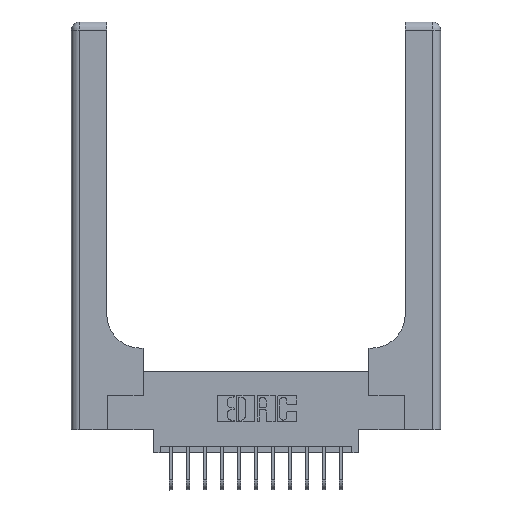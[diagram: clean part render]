
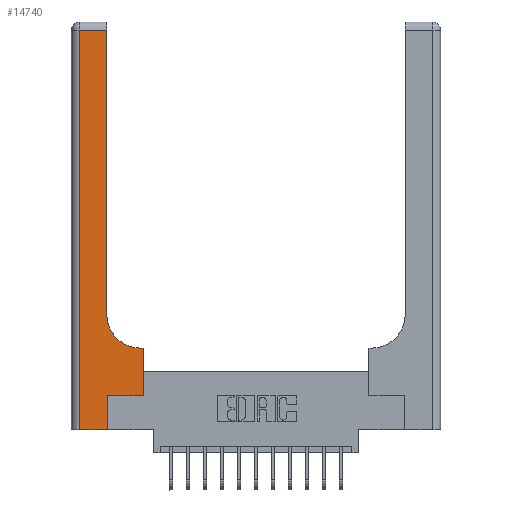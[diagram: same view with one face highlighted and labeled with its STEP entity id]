
A CAD part, top view. The second image highlights one B-rep face of the part: STEP entity #14740.
In plain terms, the highlighted planar face has unit normal (0, 0, 1).
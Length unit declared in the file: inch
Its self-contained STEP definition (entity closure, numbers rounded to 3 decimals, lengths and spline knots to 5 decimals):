
#79 = DIRECTION ( 'NONE',  ( 1., 0., 0. ) ) ;
#195 = VERTEX_POINT ( 'NONE', #12885 ) ;
#504 = CARTESIAN_POINT ( 'NONE',  ( 0.06, 3., 0.37 ) ) ;
#670 = CIRCLE ( 'NONE', #18062, 0.25 ) ;
#722 = VERTEX_POINT ( 'NONE', #9341 ) ;
#1000 = CARTESIAN_POINT ( 'NONE',  ( 0.51, 0.85, 0.37 ) ) ;
#1031 = DIRECTION ( 'NONE',  ( 0., 0., -1. ) ) ;
#1051 = LINE ( 'NONE', #11383, #17765 ) ;
#1323 = DIRECTION ( 'NONE',  ( 0., 1., 0. ) ) ;
#1368 = DIRECTION ( 'NONE',  ( 0., 0., -1. ) ) ;
#1375 = EDGE_CURVE ( 'NONE', #17372, #10682, #7767, .T. ) ;
#1478 = ORIENTED_EDGE ( 'NONE', *, *, #1375, .T. ) ;
#2265 = PLANE ( 'NONE',  #11930 ) ;
#2561 = ORIENTED_EDGE ( 'NONE', *, *, #18293, .T. ) ;
#2565 = CARTESIAN_POINT ( 'NONE',  ( 0.26, 3., 0.37 ) ) ;
#2668 = CARTESIAN_POINT ( 'NONE',  ( 0.265, 0., 0.37 ) ) ;
#2794 = CARTESIAN_POINT ( 'NONE',  ( 0.06, 2.94, 0.37 ) ) ;
#3109 = EDGE_CURVE ( 'NONE', #13241, #4829, #8973, .T. ) ;
#3165 = DIRECTION ( 'NONE',  ( -1., 0., 0. ) ) ;
#3443 = ORIENTED_EDGE ( 'NONE', *, *, #16912, .T. ) ;
#3527 = FACE_OUTER_BOUND ( 'NONE', #12988, .T. ) ;
#4707 = EDGE_CURVE ( 'NONE', #9349, #17372, #6609, .T. ) ;
#4770 = VERTEX_POINT ( 'NONE', #13927 ) ;
#4829 = VERTEX_POINT ( 'NONE', #18791 ) ;
#4986 = ORIENTED_EDGE ( 'NONE', *, *, #4707, .T. ) ;
#6500 = DIRECTION ( 'NONE',  ( -1., 0., 0. ) ) ;
#6508 = CARTESIAN_POINT ( 'NONE',  ( 0.265, 0., 0.37 ) ) ;
#6609 = LINE ( 'NONE', #2565, #9350 ) ;
#6791 = CARTESIAN_POINT ( 'NONE',  ( 0., 3., 0.37 ) ) ;
#7500 = CARTESIAN_POINT ( 'NONE',  ( 0.265, 0.25, 0.37 ) ) ;
#7767 = LINE ( 'NONE', #16255, #10397 ) ;
#7913 = CARTESIAN_POINT ( 'NONE',  ( 0., 0., 0.37 ) ) ;
#8245 = CARTESIAN_POINT ( 'NONE',  ( 0.26, 0.85, 0.37 ) ) ;
#8683 = LINE ( 'NONE', #6508, #18330 ) ;
#8973 = LINE ( 'NONE', #11668, #12826 ) ;
#9188 = ORIENTED_EDGE ( 'NONE', *, *, #16357, .T. ) ;
#9341 = CARTESIAN_POINT ( 'NONE',  ( 0.06, 0., 0.37 ) ) ;
#9349 = VERTEX_POINT ( 'NONE', #8245 ) ;
#9350 = VECTOR ( 'NONE', #17087, 39.37008 ) ;
#9550 = DIRECTION ( 'NONE',  ( 0., 1., 0. ) ) ;
#9729 = DIRECTION ( 'NONE',  ( 1., 0., 0. ) ) ;
#9775 = ORIENTED_EDGE ( 'NONE', *, *, #14825, .T. ) ;
#9786 = EDGE_CURVE ( 'NONE', #195, #4770, #13342, .T. ) ;
#10045 = VECTOR ( 'NONE', #17557, 39.37008 ) ;
#10397 = VECTOR ( 'NONE', #3165, 39.37008 ) ;
#10682 = VERTEX_POINT ( 'NONE', #2794 ) ;
#10752 = LINE ( 'NONE', #504, #17469 ) ;
#10783 = LINE ( 'NONE', #7913, #15305 ) ;
#11383 = CARTESIAN_POINT ( 'NONE',  ( 0.528, 0.25, 0.37 ) ) ;
#11668 = CARTESIAN_POINT ( 'NONE',  ( 0.265, 0.25, 0.37 ) ) ;
#11930 = AXIS2_PLACEMENT_3D ( 'NONE', #6791, #1031, #6500 ) ;
#12074 = CARTESIAN_POINT ( 'NONE',  ( 0.26, 2.94, 0.37 ) ) ;
#12739 = ORIENTED_EDGE ( 'NONE', *, *, #3109, .T. ) ;
#12826 = VECTOR ( 'NONE', #79, 39.37008 ) ;
#12885 = CARTESIAN_POINT ( 'NONE',  ( 0.528, 0.6, 0.37 ) ) ;
#12988 = EDGE_LOOP ( 'NONE', ( #4986, #1478, #3443, #15955, #9775, #12739, #9188, #15286, #2561 ) ) ;
#13241 = VERTEX_POINT ( 'NONE', #7500 ) ;
#13342 = LINE ( 'NONE', #16218, #10045 ) ;
#13883 = DIRECTION ( 'NONE',  ( 0., -1., 0. ) ) ;
#13927 = CARTESIAN_POINT ( 'NONE',  ( 0.51, 0.6, 0.37 ) ) ;
#14740 = ADVANCED_FACE ( 'NONE', ( #3527 ), #2265, .F. ) ;
#14825 = EDGE_CURVE ( 'NONE', #16240, #13241, #8683, .T. ) ;
#15286 = ORIENTED_EDGE ( 'NONE', *, *, #9786, .T. ) ;
#15305 = VECTOR ( 'NONE', #9729, 39.37008 ) ;
#15955 = ORIENTED_EDGE ( 'NONE', *, *, #17792, .T. ) ;
#16218 = CARTESIAN_POINT ( 'NONE',  ( 0.26, 0.6, 0.37 ) ) ;
#16240 = VERTEX_POINT ( 'NONE', #2668 ) ;
#16255 = CARTESIAN_POINT ( 'NONE',  ( 0., 2.94, 0.37 ) ) ;
#16357 = EDGE_CURVE ( 'NONE', #4829, #195, #1051, .T. ) ;
#16912 = EDGE_CURVE ( 'NONE', #10682, #722, #10752, .T. ) ;
#17087 = DIRECTION ( 'NONE',  ( 0., 1., 0. ) ) ;
#17372 = VERTEX_POINT ( 'NONE', #12074 ) ;
#17469 = VECTOR ( 'NONE', #13883, 39.37008 ) ;
#17557 = DIRECTION ( 'NONE',  ( -1., 0., 0. ) ) ;
#17765 = VECTOR ( 'NONE', #1323, 39.37008 ) ;
#17792 = EDGE_CURVE ( 'NONE', #722, #16240, #10783, .T. ) ;
#18062 = AXIS2_PLACEMENT_3D ( 'NONE', #1000, #1368, #18478 ) ;
#18293 = EDGE_CURVE ( 'NONE', #4770, #9349, #670, .T. ) ;
#18330 = VECTOR ( 'NONE', #9550, 39.37008 ) ;
#18478 = DIRECTION ( 'NONE',  ( 1., 0., 0. ) ) ;
#18791 = CARTESIAN_POINT ( 'NONE',  ( 0.528, 0.25, 0.37 ) ) ;
